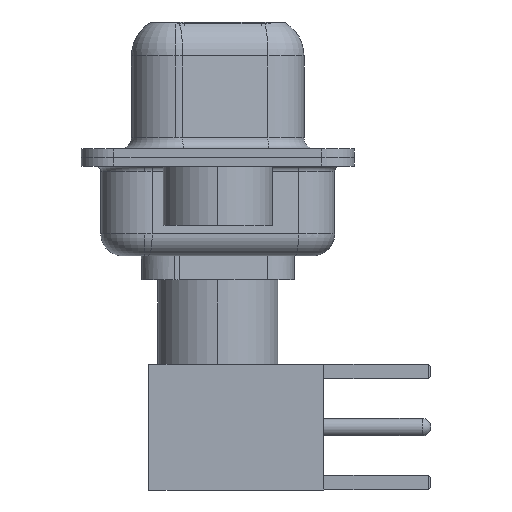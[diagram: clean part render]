
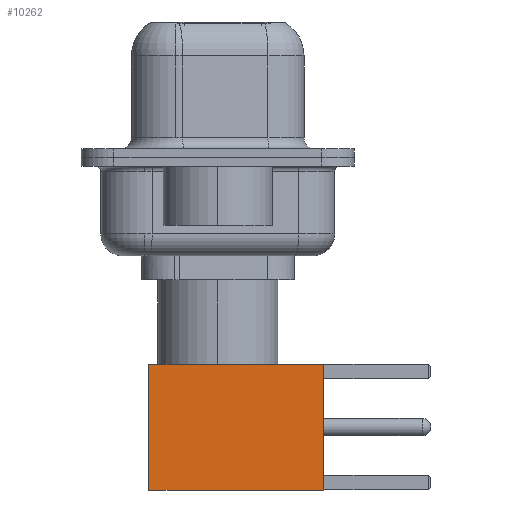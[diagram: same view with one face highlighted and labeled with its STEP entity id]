
A CAD part, left-side view. The second image highlights one B-rep face of the part: STEP entity #10262.
In plain terms, the highlighted face is planar.
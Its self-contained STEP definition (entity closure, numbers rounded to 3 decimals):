
#167 = ORIENTED_EDGE ( 'NONE', *, *, #2626, .T. ) ;
#389 = VERTEX_POINT ( 'NONE', #11580 ) ;
#436 = CARTESIAN_POINT ( 'NONE',  ( -2.875, 2.875, 0. ) ) ;
#1235 = ORIENTED_EDGE ( 'NONE', *, *, #3246, .F. ) ;
#1459 = PLANE ( 'NONE',  #14199 ) ;
#1601 = LINE ( 'NONE', #3354, #13908 ) ;
#1890 = CARTESIAN_POINT ( 'NONE',  ( 2.875, 2.875, 0. ) ) ;
#2240 = VERTEX_POINT ( 'NONE', #436 ) ;
#2394 = EDGE_CURVE ( 'NONE', #15698, #2240, #19022, .T. ) ;
#2626 = EDGE_CURVE ( 'NONE', #389, #17262, #16870, .T. ) ;
#3246 = EDGE_CURVE ( 'NONE', #389, #15698, #18883, .T. ) ;
#3354 = CARTESIAN_POINT ( 'NONE',  ( 0., 2.875, 0. ) ) ;
#3811 = CARTESIAN_POINT ( 'NONE',  ( 0., 2.875, 8. ) ) ;
#6883 = CARTESIAN_POINT ( 'NONE',  ( -2.875, 2.875, 0. ) ) ;
#7413 = DIRECTION ( 'NONE',  ( 0., 1., 0. ) ) ;
#7774 = EDGE_LOOP ( 'NONE', ( #167, #16788, #9951, #1235 ) ) ;
#8822 = VECTOR ( 'NONE', #15869, 1000. ) ;
#8961 = CARTESIAN_POINT ( 'NONE',  ( 2.875, 2.875, 0. ) ) ;
#9951 = ORIENTED_EDGE ( 'NONE', *, *, #2394, .F. ) ;
#10262 = ADVANCED_FACE ( 'NONE', ( #16245 ), #1459, .T. ) ;
#10746 = EDGE_CURVE ( 'NONE', #17262, #2240, #1601, .T. ) ;
#11133 = DIRECTION ( 'NONE',  ( 0., 0., -1. ) ) ;
#11580 = CARTESIAN_POINT ( 'NONE',  ( 2.875, 2.875, 8. ) ) ;
#12845 = VECTOR ( 'NONE', #11133, 1000. ) ;
#13330 = DIRECTION ( 'NONE',  ( 0., 0., 1. ) ) ;
#13908 = VECTOR ( 'NONE', #18330, 1000. ) ;
#14199 = AXIS2_PLACEMENT_3D ( 'NONE', #8961, #7413, #13330 ) ;
#15698 = VERTEX_POINT ( 'NONE', #16438 ) ;
#15869 = DIRECTION ( 'NONE',  ( -1., 0., 0. ) ) ;
#16245 = FACE_OUTER_BOUND ( 'NONE', #7774, .T. ) ;
#16438 = CARTESIAN_POINT ( 'NONE',  ( -2.875, 2.875, 8. ) ) ;
#16788 = ORIENTED_EDGE ( 'NONE', *, *, #10746, .T. ) ;
#16870 = LINE ( 'NONE', #1890, #12845 ) ;
#17262 = VERTEX_POINT ( 'NONE', #18475 ) ;
#17559 = DIRECTION ( 'NONE',  ( 0., 0., -1. ) ) ;
#18330 = DIRECTION ( 'NONE',  ( -1., 0., 0. ) ) ;
#18475 = CARTESIAN_POINT ( 'NONE',  ( 2.875, 2.875, 0. ) ) ;
#18883 = LINE ( 'NONE', #3811, #8822 ) ;
#19022 = LINE ( 'NONE', #6883, #19038 ) ;
#19038 = VECTOR ( 'NONE', #17559, 1000. ) ;
